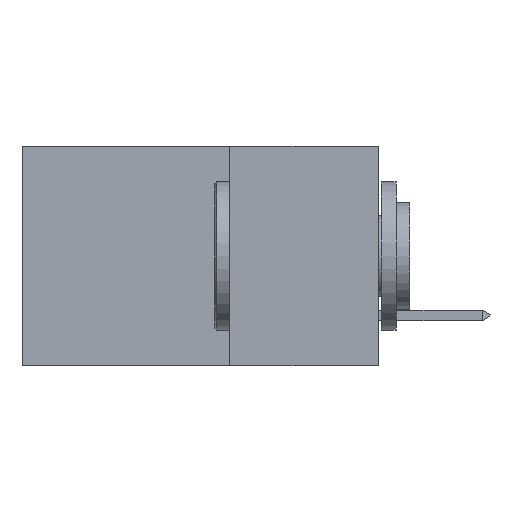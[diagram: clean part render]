
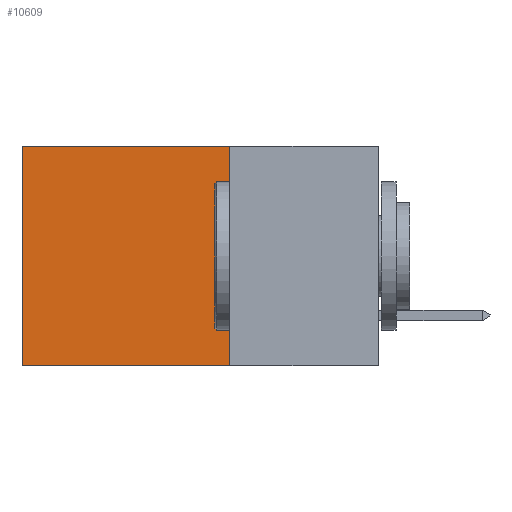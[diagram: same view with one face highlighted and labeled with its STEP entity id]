
A CAD part, left-side view. The second image highlights one B-rep face of the part: STEP entity #10609.
In plain terms, the highlighted planar face has unit normal (-1, 0, 0).
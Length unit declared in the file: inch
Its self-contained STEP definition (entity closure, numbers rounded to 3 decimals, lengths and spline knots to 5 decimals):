
#445 = AXIS2_PLACEMENT_3D ( 'NONE', #931, #10965, #10901 ) ;
#931 = CARTESIAN_POINT ( 'NONE',  ( 0.2615, 0.25, -0.37 ) ) ;
#1006 = CARTESIAN_POINT ( 'NONE',  ( 0.2615, 0.25, -0.37 ) ) ;
#1373 = CARTESIAN_POINT ( 'NONE',  ( 0.2615, 0.25, -0.37 ) ) ;
#2049 = LINE ( 'NONE', #5129, #10161 ) ;
#2642 = EDGE_CURVE ( 'NONE', #6939, #5055, #2854, .T. ) ;
#2854 = LINE ( 'NONE', #1006, #10535 ) ;
#2870 = CARTESIAN_POINT ( 'NONE',  ( 0.2615, 0.25, -0.37 ) ) ;
#2989 = CARTESIAN_POINT ( 'NONE',  ( 0.2615, 0.25, 0. ) ) ;
#3040 = ORIENTED_EDGE ( 'NONE', *, *, #3627, .T. ) ;
#3627 = EDGE_CURVE ( 'NONE', #11238, #6100, #2049, .T. ) ;
#5055 = VERTEX_POINT ( 'NONE', #1373 ) ;
#5129 = CARTESIAN_POINT ( 'NONE',  ( 0.2615, 0.6, -0.37 ) ) ;
#5587 = LINE ( 'NONE', #6555, #12183 ) ;
#5992 = CARTESIAN_POINT ( 'NONE',  ( 0.2615, 0.6, 0. ) ) ;
#6100 = VERTEX_POINT ( 'NONE', #9218 ) ;
#6555 = CARTESIAN_POINT ( 'NONE',  ( 0.2615, 0.25, 0. ) ) ;
#6834 = FACE_OUTER_BOUND ( 'NONE', #8933, .T. ) ;
#6939 = VERTEX_POINT ( 'NONE', #2989 ) ;
#7591 = EDGE_CURVE ( 'NONE', #6939, #11238, #5587, .T. ) ;
#8532 = ORIENTED_EDGE ( 'NONE', *, *, #2642, .F. ) ;
#8933 = EDGE_LOOP ( 'NONE', ( #3040, #10975, #8532, #9548 ) ) ;
#9218 = CARTESIAN_POINT ( 'NONE',  ( 0.2615, 0.6, -0.37 ) ) ;
#9479 = VECTOR ( 'NONE', #10868, 39.37008 ) ;
#9548 = ORIENTED_EDGE ( 'NONE', *, *, #7591, .T. ) ;
#10038 = DIRECTION ( 'NONE',  ( 0., 0., -1. ) ) ;
#10161 = VECTOR ( 'NONE', #10038, 39.37008 ) ;
#10535 = VECTOR ( 'NONE', #12675, 39.37008 ) ;
#10557 = DIRECTION ( 'NONE',  ( 0., 1., 0. ) ) ;
#10609 = ADVANCED_FACE ( 'NONE', ( #6834 ), #11874, .F. ) ;
#10868 = DIRECTION ( 'NONE',  ( 0., 1., 0. ) ) ;
#10901 = DIRECTION ( 'NONE',  ( 0., 0., -1. ) ) ;
#10965 = DIRECTION ( 'NONE',  ( 1., 0., 0. ) ) ;
#10975 = ORIENTED_EDGE ( 'NONE', *, *, #11514, .F. ) ;
#11238 = VERTEX_POINT ( 'NONE', #5992 ) ;
#11514 = EDGE_CURVE ( 'NONE', #5055, #6100, #12819, .T. ) ;
#11874 = PLANE ( 'NONE',  #445 ) ;
#12183 = VECTOR ( 'NONE', #10557, 39.37008 ) ;
#12675 = DIRECTION ( 'NONE',  ( 0., 0., -1. ) ) ;
#12819 = LINE ( 'NONE', #2870, #9479 ) ;
